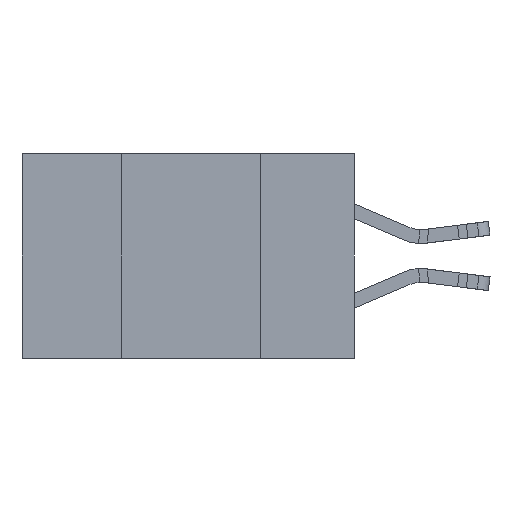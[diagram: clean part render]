
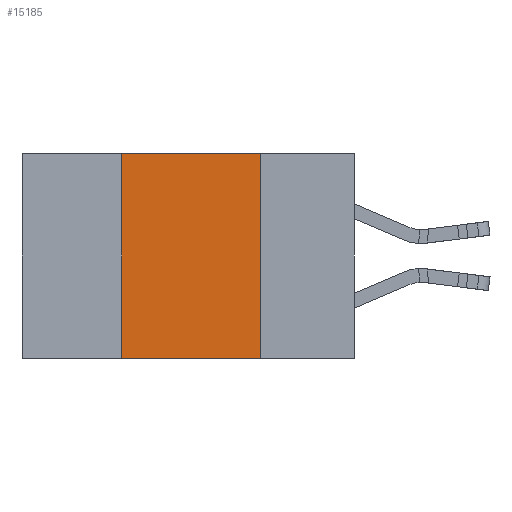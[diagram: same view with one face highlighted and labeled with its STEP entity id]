
A CAD part, left-side view. The second image highlights one B-rep face of the part: STEP entity #15185.
In plain terms, the highlighted planar face has unit normal (-1, 0, 0).
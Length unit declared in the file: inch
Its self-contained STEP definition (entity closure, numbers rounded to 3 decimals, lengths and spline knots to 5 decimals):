
#2230 = VECTOR ( 'NONE', #4568, 39.37008 ) ;
#2756 = EDGE_CURVE ( 'NONE', #21055, #22623, #24416, .T. ) ;
#3426 = CARTESIAN_POINT ( 'NONE',  ( 0., 0.17, -0.37 ) ) ;
#3583 = CARTESIAN_POINT ( 'NONE',  ( 0., 0.42, -0.37 ) ) ;
#4515 = ORIENTED_EDGE ( 'NONE', *, *, #16574, .F. ) ;
#4568 = DIRECTION ( 'NONE',  ( 0., -1., 0. ) ) ;
#5053 = LINE ( 'NONE', #3426, #9633 ) ;
#6012 = ORIENTED_EDGE ( 'NONE', *, *, #2756, .F. ) ;
#6030 = LINE ( 'NONE', #23779, #15734 ) ;
#6303 = CARTESIAN_POINT ( 'NONE',  ( 0., 0.42, 0. ) ) ;
#6381 = DIRECTION ( 'NONE',  ( 0., -1., 0. ) ) ;
#6556 = VERTEX_POINT ( 'NONE', #3583 ) ;
#7749 = AXIS2_PLACEMENT_3D ( 'NONE', #20647, #9121, #22562 ) ;
#8582 = CARTESIAN_POINT ( 'NONE',  ( 0., 0.17, 0. ) ) ;
#9121 = DIRECTION ( 'NONE',  ( 1., 0., 0. ) ) ;
#9633 = VECTOR ( 'NONE', #17008, 39.37008 ) ;
#13938 = ORIENTED_EDGE ( 'NONE', *, *, #14956, .T. ) ;
#14486 = EDGE_LOOP ( 'NONE', ( #4515, #6012, #19040, #13938 ) ) ;
#14956 = EDGE_CURVE ( 'NONE', #6556, #21665, #6030, .T. ) ;
#15185 = ADVANCED_FACE ( 'NONE', ( #24921 ), #16790, .F. ) ;
#15734 = VECTOR ( 'NONE', #6381, 39.37008 ) ;
#16574 = EDGE_CURVE ( 'NONE', #22623, #21665, #5053, .T. ) ;
#16790 = PLANE ( 'NONE',  #7749 ) ;
#17008 = DIRECTION ( 'NONE',  ( 0., 0., -1. ) ) ;
#17552 = EDGE_CURVE ( 'NONE', #6556, #21055, #23406, .T. ) ;
#17558 = CARTESIAN_POINT ( 'NONE',  ( 0., 0.42, -0.37 ) ) ;
#17644 = CARTESIAN_POINT ( 'NONE',  ( 0., 0.17, -0.37 ) ) ;
#18974 = VECTOR ( 'NONE', #21478, 39.37008 ) ;
#19040 = ORIENTED_EDGE ( 'NONE', *, *, #17552, .F. ) ;
#20647 = CARTESIAN_POINT ( 'NONE',  ( 0., 0.6, 0. ) ) ;
#21055 = VERTEX_POINT ( 'NONE', #6303 ) ;
#21478 = DIRECTION ( 'NONE',  ( 0., 0., 1. ) ) ;
#21665 = VERTEX_POINT ( 'NONE', #17644 ) ;
#22562 = DIRECTION ( 'NONE',  ( 0., 0., -1. ) ) ;
#22623 = VERTEX_POINT ( 'NONE', #8582 ) ;
#23369 = CARTESIAN_POINT ( 'NONE',  ( 0., 0.6, 0. ) ) ;
#23406 = LINE ( 'NONE', #17558, #18974 ) ;
#23779 = CARTESIAN_POINT ( 'NONE',  ( 0., 0.6, -0.37 ) ) ;
#24416 = LINE ( 'NONE', #23369, #2230 ) ;
#24921 = FACE_OUTER_BOUND ( 'NONE', #14486, .T. ) ;
